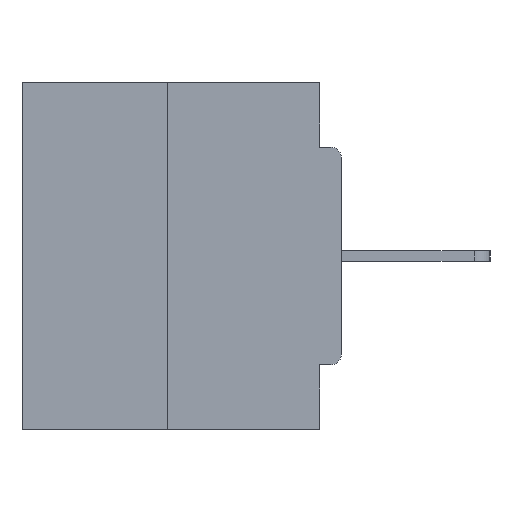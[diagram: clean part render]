
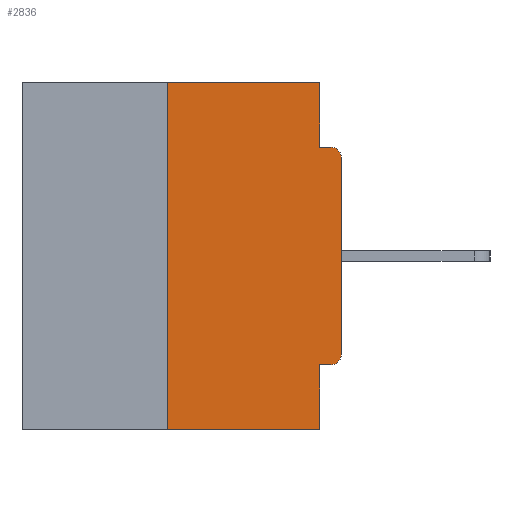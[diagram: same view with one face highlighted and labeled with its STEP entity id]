
A CAD part, left-side view. The second image highlights one B-rep face of the part: STEP entity #2836.
In plain terms, the highlighted planar face has unit normal (-1, 0, 0).
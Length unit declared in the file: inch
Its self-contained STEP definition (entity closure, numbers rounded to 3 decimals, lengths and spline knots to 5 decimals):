
#435 = DIRECTION ( 'NONE',  ( 0., 0., -1. ) ) ;
#570 = DIRECTION ( 'NONE',  ( 1., 0., 0. ) ) ;
#1686 = VERTEX_POINT ( 'NONE', #20563 ) ;
#2052 = ORIENTED_EDGE ( 'NONE', *, *, #21171, .T. ) ;
#2300 = CARTESIAN_POINT ( 'NONE',  ( 0., 0.031, -0.0935 ) ) ;
#2376 = VECTOR ( 'NONE', #16491, 39.37008 ) ;
#2611 = CARTESIAN_POINT ( 'NONE',  ( 0., 0.015, -0.3915 ) ) ;
#2836 = ADVANCED_FACE ( 'NONE', ( #12162 ), #6975, .F. ) ;
#3032 = EDGE_CURVE ( 'NONE', #3517, #6647, #31045, .T. ) ;
#3517 = VERTEX_POINT ( 'NONE', #20983 ) ;
#3703 = EDGE_CURVE ( 'NONE', #17383, #26545, #19423, .T. ) ;
#3767 = LINE ( 'NONE', #5987, #23371 ) ;
#3842 = CARTESIAN_POINT ( 'NONE',  ( 0., 0.46, -0.5 ) ) ;
#3946 = DIRECTION ( 'NONE',  ( 0., -1., 0. ) ) ;
#5255 = VERTEX_POINT ( 'NONE', #18764 ) ;
#5274 = CARTESIAN_POINT ( 'NONE',  ( 0., 0.46, 0. ) ) ;
#5463 = DIRECTION ( 'NONE',  ( 0., 0., -1. ) ) ;
#5724 = EDGE_CURVE ( 'NONE', #5255, #24116, #29834, .T. ) ;
#5772 = EDGE_CURVE ( 'NONE', #26545, #27947, #8902, .T. ) ;
#5987 = CARTESIAN_POINT ( 'NONE',  ( 0., 0., -0.4065 ) ) ;
#6647 = VERTEX_POINT ( 'NONE', #2300 ) ;
#6975 = PLANE ( 'NONE',  #29822 ) ;
#7636 = ORIENTED_EDGE ( 'NONE', *, *, #22868, .F. ) ;
#7989 = CARTESIAN_POINT ( 'NONE',  ( 0., 0.25, 0. ) ) ;
#8902 = LINE ( 'NONE', #22586, #2376 ) ;
#9456 = CARTESIAN_POINT ( 'NONE',  ( 0., 0., -0.3915 ) ) ;
#10394 = LINE ( 'NONE', #17636, #15361 ) ;
#10441 = LINE ( 'NONE', #5274, #29092 ) ;
#10463 = CARTESIAN_POINT ( 'NONE',  ( 0., 0.015, -0.1085 ) ) ;
#10472 = VECTOR ( 'NONE', #30612, 39.37008 ) ;
#11667 = ORIENTED_EDGE ( 'NONE', *, *, #25097, .F. ) ;
#11743 = VECTOR ( 'NONE', #15577, 39.37008 ) ;
#12162 = FACE_OUTER_BOUND ( 'NONE', #19438, .T. ) ;
#12164 = AXIS2_PLACEMENT_3D ( 'NONE', #10463, #27525, #12917 ) ;
#12917 = DIRECTION ( 'NONE',  ( 0., 0., -1. ) ) ;
#12925 = EDGE_CURVE ( 'NONE', #1686, #14193, #10394, .T. ) ;
#13273 = ORIENTED_EDGE ( 'NONE', *, *, #3703, .T. ) ;
#13307 = DIRECTION ( 'NONE',  ( 0., 1., 0. ) ) ;
#14193 = VERTEX_POINT ( 'NONE', #25316 ) ;
#15361 = VECTOR ( 'NONE', #5463, 39.37008 ) ;
#15518 = ORIENTED_EDGE ( 'NONE', *, *, #5724, .F. ) ;
#15577 = DIRECTION ( 'NONE',  ( 0., 0., -1. ) ) ;
#15838 = CARTESIAN_POINT ( 'NONE',  ( 0., 0.015, -0.4065 ) ) ;
#16038 = CARTESIAN_POINT ( 'NONE',  ( 0., 0.031, 0. ) ) ;
#16277 = ORIENTED_EDGE ( 'NONE', *, *, #28396, .F. ) ;
#16491 = DIRECTION ( 'NONE',  ( 0., 0., 1. ) ) ;
#16848 = VECTOR ( 'NONE', #30403, 39.37008 ) ;
#17383 = VERTEX_POINT ( 'NONE', #15838 ) ;
#17636 = CARTESIAN_POINT ( 'NONE',  ( 0., 0.031, -0.5 ) ) ;
#18402 = LINE ( 'NONE', #28082, #16848 ) ;
#18753 = VERTEX_POINT ( 'NONE', #27699 ) ;
#18764 = CARTESIAN_POINT ( 'NONE',  ( 0., 0.25, -0.5 ) ) ;
#19334 = CIRCLE ( 'NONE', #12164, 0.015 ) ;
#19423 = CIRCLE ( 'NONE', #21637, 0.015 ) ;
#19438 = EDGE_LOOP ( 'NONE', ( #16277, #15518, #2052, #29909, #7636, #13273, #27764, #26214, #11667, #30219 ) ) ;
#19990 = DIRECTION ( 'NONE',  ( 0., -1., 0. ) ) ;
#20410 = VECTOR ( 'NONE', #3946, 39.37008 ) ;
#20534 = CARTESIAN_POINT ( 'NONE',  ( 0., 0.46, 0. ) ) ;
#20563 = CARTESIAN_POINT ( 'NONE',  ( 0., 0.031, -0.4065 ) ) ;
#20983 = CARTESIAN_POINT ( 'NONE',  ( 0., 0.031, 0. ) ) ;
#21171 = EDGE_CURVE ( 'NONE', #5255, #14193, #26878, .T. ) ;
#21524 = CARTESIAN_POINT ( 'NONE',  ( 0., 0.25, 0. ) ) ;
#21637 = AXIS2_PLACEMENT_3D ( 'NONE', #2611, #27097, #30314 ) ;
#22586 = CARTESIAN_POINT ( 'NONE',  ( 0., 0., 0. ) ) ;
#22868 = EDGE_CURVE ( 'NONE', #17383, #1686, #3767, .T. ) ;
#23371 = VECTOR ( 'NONE', #13307, 39.37008 ) ;
#24116 = VERTEX_POINT ( 'NONE', #21524 ) ;
#25097 = EDGE_CURVE ( 'NONE', #6647, #18753, #18402, .T. ) ;
#25316 = CARTESIAN_POINT ( 'NONE',  ( 0., 0.031, -0.5 ) ) ;
#25534 = CARTESIAN_POINT ( 'NONE',  ( 0., 0., -0.1085 ) ) ;
#26214 = ORIENTED_EDGE ( 'NONE', *, *, #27849, .T. ) ;
#26545 = VERTEX_POINT ( 'NONE', #9456 ) ;
#26878 = LINE ( 'NONE', #3842, #20410 ) ;
#27097 = DIRECTION ( 'NONE',  ( -1., 0., 0. ) ) ;
#27525 = DIRECTION ( 'NONE',  ( -1., 0., 0. ) ) ;
#27699 = CARTESIAN_POINT ( 'NONE',  ( 0., 0.015, -0.0935 ) ) ;
#27764 = ORIENTED_EDGE ( 'NONE', *, *, #5772, .T. ) ;
#27849 = EDGE_CURVE ( 'NONE', #27947, #18753, #19334, .T. ) ;
#27947 = VERTEX_POINT ( 'NONE', #25534 ) ;
#28082 = CARTESIAN_POINT ( 'NONE',  ( 0., 0., -0.0935 ) ) ;
#28396 = EDGE_CURVE ( 'NONE', #24116, #3517, #10441, .T. ) ;
#29092 = VECTOR ( 'NONE', #19990, 39.37008 ) ;
#29822 = AXIS2_PLACEMENT_3D ( 'NONE', #20534, #570, #435 ) ;
#29834 = LINE ( 'NONE', #7989, #10472 ) ;
#29909 = ORIENTED_EDGE ( 'NONE', *, *, #12925, .F. ) ;
#30219 = ORIENTED_EDGE ( 'NONE', *, *, #3032, .F. ) ;
#30314 = DIRECTION ( 'NONE',  ( 0., 0., -1. ) ) ;
#30403 = DIRECTION ( 'NONE',  ( 0., -1., 0. ) ) ;
#30612 = DIRECTION ( 'NONE',  ( 0., 0., 1. ) ) ;
#31045 = LINE ( 'NONE', #16038, #11743 ) ;
